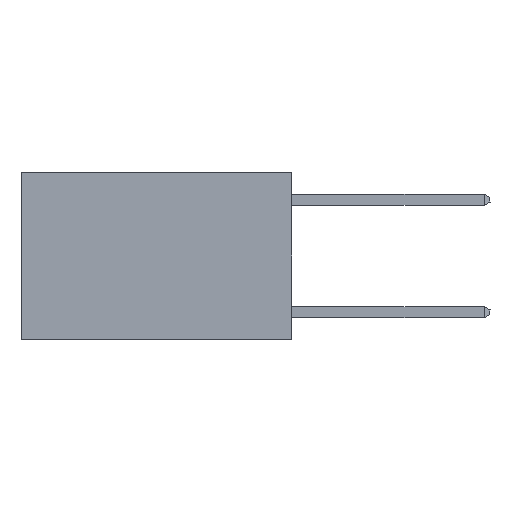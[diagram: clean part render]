
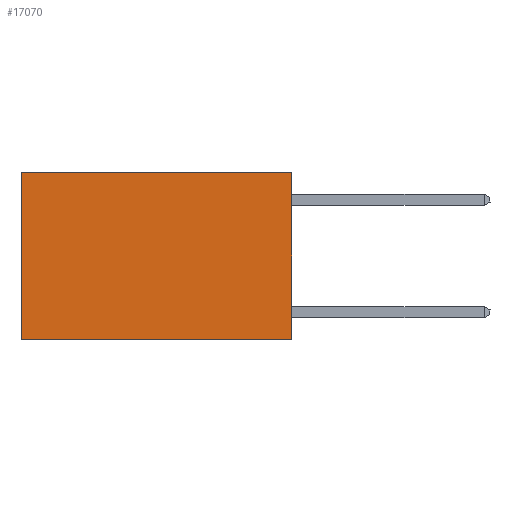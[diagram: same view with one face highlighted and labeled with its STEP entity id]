
A CAD part, left-side view. The second image highlights one B-rep face of the part: STEP entity #17070.
In plain terms, the highlighted planar face has unit normal (-1, 0, 0).
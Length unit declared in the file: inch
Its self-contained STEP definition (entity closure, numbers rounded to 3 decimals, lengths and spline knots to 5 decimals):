
#892 = VECTOR ( 'NONE', #2661, 39.37008 ) ;
#1190 = CARTESIAN_POINT ( 'NONE',  ( 0.2625, 0.6, 0. ) ) ;
#1899 = DIRECTION ( 'NONE',  ( 0., 1., 0. ) ) ;
#2091 = DIRECTION ( 'NONE',  ( 1., 0., 0. ) ) ;
#2384 = CARTESIAN_POINT ( 'NONE',  ( 0.2625, 0., 0. ) ) ;
#2661 = DIRECTION ( 'NONE',  ( 0., 1., 0. ) ) ;
#3231 = LINE ( 'NONE', #5017, #5591 ) ;
#3923 = CARTESIAN_POINT ( 'NONE',  ( 0.2625, 0., 0. ) ) ;
#5017 = CARTESIAN_POINT ( 'NONE',  ( 0.2625, 0.6, 0. ) ) ;
#5453 = EDGE_CURVE ( 'NONE', #12512, #11492, #28516, .T. ) ;
#5591 = VECTOR ( 'NONE', #23099, 39.37008 ) ;
#6672 = ORIENTED_EDGE ( 'NONE', *, *, #8038, .T. ) ;
#7144 = DIRECTION ( 'NONE',  ( 0., 0., -1. ) ) ;
#7629 = ORIENTED_EDGE ( 'NONE', *, *, #5453, .F. ) ;
#8038 = EDGE_CURVE ( 'NONE', #25152, #8819, #3231, .T. ) ;
#8819 = VERTEX_POINT ( 'NONE', #23477 ) ;
#9322 = CARTESIAN_POINT ( 'NONE',  ( 0.2625, 0., -0.37 ) ) ;
#11298 = PLANE ( 'NONE',  #18572 ) ;
#11492 = VERTEX_POINT ( 'NONE', #9322 ) ;
#12309 = CARTESIAN_POINT ( 'NONE',  ( 0.2625, 0., 0. ) ) ;
#12348 = CARTESIAN_POINT ( 'NONE',  ( 0.2625, 0., -0.37 ) ) ;
#12512 = VERTEX_POINT ( 'NONE', #12309 ) ;
#14384 = CARTESIAN_POINT ( 'NONE',  ( 0.2625, 0., 0. ) ) ;
#15469 = DIRECTION ( 'NONE',  ( 0., 0., -1. ) ) ;
#15614 = VECTOR ( 'NONE', #1899, 39.37008 ) ;
#17070 = ADVANCED_FACE ( 'NONE', ( #20486 ), #11298, .F. ) ;
#17831 = EDGE_LOOP ( 'NONE', ( #6672, #21201, #7629, #24159 ) ) ;
#17900 = LINE ( 'NONE', #12348, #15614 ) ;
#18572 = AXIS2_PLACEMENT_3D ( 'NONE', #2384, #2091, #7144 ) ;
#20486 = FACE_OUTER_BOUND ( 'NONE', #17831, .T. ) ;
#21201 = ORIENTED_EDGE ( 'NONE', *, *, #27936, .F. ) ;
#22964 = VECTOR ( 'NONE', #15469, 39.37008 ) ;
#23099 = DIRECTION ( 'NONE',  ( 0., 0., -1. ) ) ;
#23477 = CARTESIAN_POINT ( 'NONE',  ( 0.2625, 0.6, -0.37 ) ) ;
#24159 = ORIENTED_EDGE ( 'NONE', *, *, #27602, .T. ) ;
#25152 = VERTEX_POINT ( 'NONE', #1190 ) ;
#25780 = LINE ( 'NONE', #14384, #892 ) ;
#27602 = EDGE_CURVE ( 'NONE', #12512, #25152, #25780, .T. ) ;
#27936 = EDGE_CURVE ( 'NONE', #11492, #8819, #17900, .T. ) ;
#28516 = LINE ( 'NONE', #3923, #22964 ) ;
